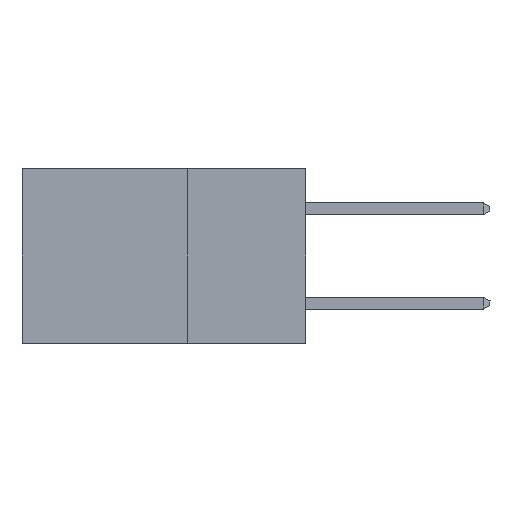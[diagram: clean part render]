
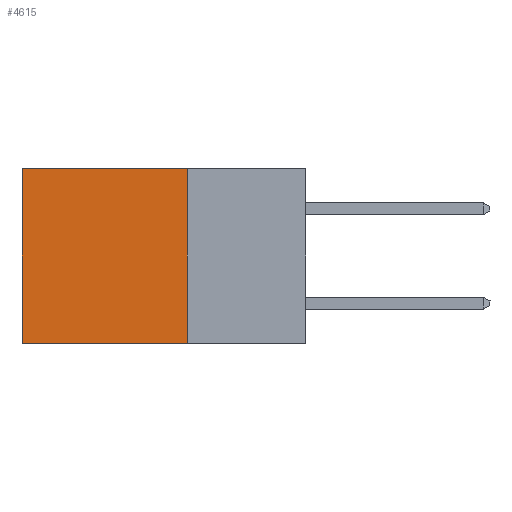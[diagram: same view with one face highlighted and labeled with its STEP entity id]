
A CAD part, left-side view. The second image highlights one B-rep face of the part: STEP entity #4615.
In plain terms, the highlighted planar face has unit normal (-1, 0, 0).
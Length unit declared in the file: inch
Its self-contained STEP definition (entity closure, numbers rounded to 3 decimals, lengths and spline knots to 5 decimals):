
#655 = CARTESIAN_POINT ( 'NONE',  ( 0.298, 0.25, -0.37 ) ) ;
#1490 = ORIENTED_EDGE ( 'NONE', *, *, #14389, .F. ) ;
#1709 = CARTESIAN_POINT ( 'NONE',  ( 0.298, 0.6, 0. ) ) ;
#2687 = CARTESIAN_POINT ( 'NONE',  ( 0.298, 0.25, 0. ) ) ;
#3234 = CARTESIAN_POINT ( 'NONE',  ( 0.298, 0.25, -0.37 ) ) ;
#3350 = ORIENTED_EDGE ( 'NONE', *, *, #3364, .F. ) ;
#3364 = EDGE_CURVE ( 'NONE', #5040, #5971, #6234, .T. ) ;
#3588 = ORIENTED_EDGE ( 'NONE', *, *, #14030, .T. ) ;
#3906 = LINE ( 'NONE', #2687, #9404 ) ;
#4615 = ADVANCED_FACE ( 'NONE', ( #6196 ), #7182, .F. ) ;
#4782 = DIRECTION ( 'NONE',  ( 1., 0., 0. ) ) ;
#5040 = VERTEX_POINT ( 'NONE', #3234 ) ;
#5473 = VECTOR ( 'NONE', #9032, 39.37008 ) ;
#5971 = VERTEX_POINT ( 'NONE', #13893 ) ;
#6196 = FACE_OUTER_BOUND ( 'NONE', #9207, .T. ) ;
#6234 = LINE ( 'NONE', #655, #8805 ) ;
#7033 = CARTESIAN_POINT ( 'NONE',  ( 0.298, 0.25, 0. ) ) ;
#7182 = PLANE ( 'NONE',  #8902 ) ;
#7379 = VECTOR ( 'NONE', #9692, 39.37008 ) ;
#7715 = ORIENTED_EDGE ( 'NONE', *, *, #14401, .T. ) ;
#8805 = VECTOR ( 'NONE', #9968, 39.37008 ) ;
#8902 = AXIS2_PLACEMENT_3D ( 'NONE', #7033, #4782, #14210 ) ;
#9032 = DIRECTION ( 'NONE',  ( 0., 0., -1. ) ) ;
#9207 = EDGE_LOOP ( 'NONE', ( #3588, #3350, #1490, #7715 ) ) ;
#9344 = LINE ( 'NONE', #14658, #5473 ) ;
#9404 = VECTOR ( 'NONE', #13302, 39.37008 ) ;
#9692 = DIRECTION ( 'NONE',  ( 0., 0., -1. ) ) ;
#9772 = LINE ( 'NONE', #10889, #7379 ) ;
#9968 = DIRECTION ( 'NONE',  ( 0., 1., 0. ) ) ;
#10889 = CARTESIAN_POINT ( 'NONE',  ( 0.298, 0.25, 0. ) ) ;
#11117 = CARTESIAN_POINT ( 'NONE',  ( 0.298, 0.25, 0. ) ) ;
#13148 = VERTEX_POINT ( 'NONE', #1709 ) ;
#13302 = DIRECTION ( 'NONE',  ( 0., 1., 0. ) ) ;
#13353 = VERTEX_POINT ( 'NONE', #11117 ) ;
#13893 = CARTESIAN_POINT ( 'NONE',  ( 0.298, 0.6, -0.37 ) ) ;
#14030 = EDGE_CURVE ( 'NONE', #13148, #5971, #9344, .T. ) ;
#14210 = DIRECTION ( 'NONE',  ( 0., 0., -1. ) ) ;
#14389 = EDGE_CURVE ( 'NONE', #13353, #5040, #9772, .T. ) ;
#14401 = EDGE_CURVE ( 'NONE', #13353, #13148, #3906, .T. ) ;
#14658 = CARTESIAN_POINT ( 'NONE',  ( 0.298, 0.6, 0. ) ) ;
